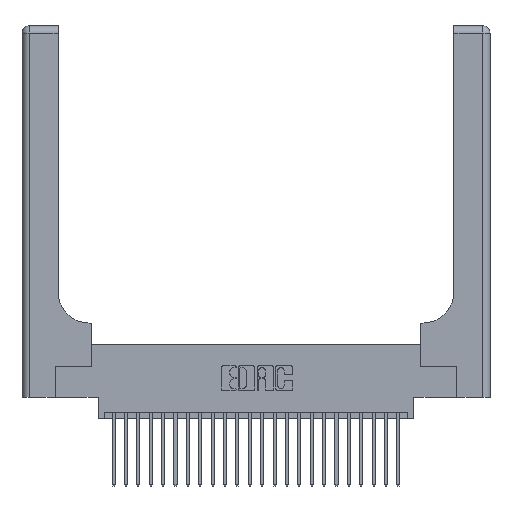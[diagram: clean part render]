
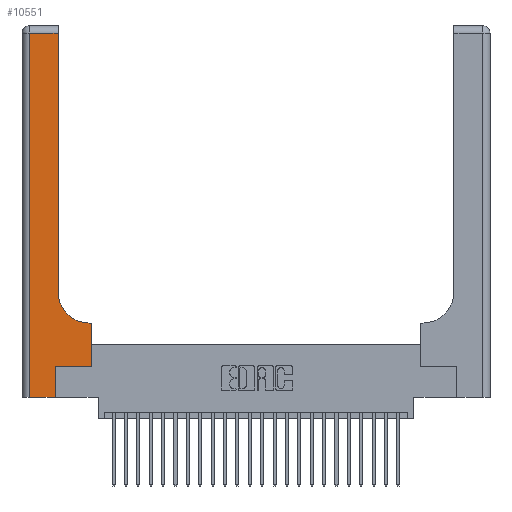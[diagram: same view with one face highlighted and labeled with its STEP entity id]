
A CAD part, top view. The second image highlights one B-rep face of the part: STEP entity #10551.
In plain terms, the highlighted planar face has unit normal (0, 0, 1).
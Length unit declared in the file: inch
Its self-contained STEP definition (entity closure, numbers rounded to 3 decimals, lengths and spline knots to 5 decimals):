
#645 = CARTESIAN_POINT ( 'NONE',  ( 0.5415, 0.6, 0.37 ) ) ;
#1730 = DIRECTION ( 'NONE',  ( 1., 0., 0. ) ) ;
#1792 = EDGE_CURVE ( 'NONE', #12622, #19311, #15619, .T. ) ;
#1806 = CARTESIAN_POINT ( 'NONE',  ( 0.269, 0., 0.37 ) ) ;
#1993 = AXIS2_PLACEMENT_3D ( 'NONE', #2356, #4441, #6528 ) ;
#2032 = EDGE_CURVE ( 'NONE', #14648, #12622, #22652, .T. ) ;
#2356 = CARTESIAN_POINT ( 'NONE',  ( 0., 3., 0.37 ) ) ;
#2486 = CARTESIAN_POINT ( 'NONE',  ( 0.5585, 0.25, 0.37 ) ) ;
#2696 = ORIENTED_EDGE ( 'NONE', *, *, #10886, .T. ) ;
#2832 = VECTOR ( 'NONE', #23845, 39.37008 ) ;
#3479 = ORIENTED_EDGE ( 'NONE', *, *, #20768, .T. ) ;
#4388 = DIRECTION ( 'NONE',  ( 0., 1., 0. ) ) ;
#4400 = LINE ( 'NONE', #2486, #14685 ) ;
#4441 = DIRECTION ( 'NONE',  ( 0., 0., -1. ) ) ;
#5413 = LINE ( 'NONE', #23519, #19540 ) ;
#5454 = CARTESIAN_POINT ( 'NONE',  ( 0., 2.94, 0.37 ) ) ;
#5510 = CARTESIAN_POINT ( 'NONE',  ( 0.06, 3., 0.37 ) ) ;
#6135 = EDGE_CURVE ( 'NONE', #19050, #14648, #14693, .T. ) ;
#6237 = EDGE_CURVE ( 'NONE', #21643, #13369, #22111, .T. ) ;
#6274 = CARTESIAN_POINT ( 'NONE',  ( 0.5585, 0.25, 0.37 ) ) ;
#6528 = DIRECTION ( 'NONE',  ( -1., 0., 0. ) ) ;
#6707 = FACE_OUTER_BOUND ( 'NONE', #12043, .T. ) ;
#7758 = EDGE_CURVE ( 'NONE', #13369, #19478, #13233, .T. ) ;
#8484 = LINE ( 'NONE', #5510, #23910 ) ;
#8554 = CARTESIAN_POINT ( 'NONE',  ( 0.2915, 2.94, 0.37 ) ) ;
#8697 = CARTESIAN_POINT ( 'NONE',  ( 0.5585, 0.6, 0.37 ) ) ;
#10245 = ORIENTED_EDGE ( 'NONE', *, *, #6135, .T. ) ;
#10497 = CARTESIAN_POINT ( 'NONE',  ( 0.06, 0., 0.37 ) ) ;
#10551 = ADVANCED_FACE ( 'NONE', ( #6707 ), #24910, .F. ) ;
#10886 = EDGE_CURVE ( 'NONE', #19478, #14336, #5413, .T. ) ;
#12017 = ORIENTED_EDGE ( 'NONE', *, *, #7758, .T. ) ;
#12043 = EDGE_LOOP ( 'NONE', ( #18715, #23758, #25726, #20669, #12017, #2696, #3479, #10245, #17749 ) ) ;
#12333 = CARTESIAN_POINT ( 'NONE',  ( 0.269, 0.25, 0.37 ) ) ;
#12622 = VERTEX_POINT ( 'NONE', #13863 ) ;
#12781 = DIRECTION ( 'NONE',  ( -1., 0., 0. ) ) ;
#12875 = CARTESIAN_POINT ( 'NONE',  ( 0.2915, 0.6, 0.37 ) ) ;
#13233 = LINE ( 'NONE', #1806, #16434 ) ;
#13369 = VERTEX_POINT ( 'NONE', #13397 ) ;
#13392 = EDGE_CURVE ( 'NONE', #20878, #21643, #8484, .T. ) ;
#13397 = CARTESIAN_POINT ( 'NONE',  ( 0.269, 0., 0.37 ) ) ;
#13863 = CARTESIAN_POINT ( 'NONE',  ( 0.2915, 0.85, 0.37 ) ) ;
#13911 = DIRECTION ( 'NONE',  ( 0., 1., 0. ) ) ;
#14336 = VERTEX_POINT ( 'NONE', #6274 ) ;
#14648 = VERTEX_POINT ( 'NONE', #645 ) ;
#14685 = VECTOR ( 'NONE', #4388, 39.37008 ) ;
#14693 = LINE ( 'NONE', #12875, #16000 ) ;
#15175 = DIRECTION ( 'NONE',  ( 0., 0., -1. ) ) ;
#15318 = CARTESIAN_POINT ( 'NONE',  ( 0., 0., 0.37 ) ) ;
#15449 = CARTESIAN_POINT ( 'NONE',  ( 0.06, 2.94, 0.37 ) ) ;
#15619 = LINE ( 'NONE', #17955, #25886 ) ;
#15639 = LINE ( 'NONE', #5454, #20754 ) ;
#16000 = VECTOR ( 'NONE', #12781, 39.37008 ) ;
#16136 = DIRECTION ( 'NONE',  ( 0., -1., 0. ) ) ;
#16434 = VECTOR ( 'NONE', #13911, 39.37008 ) ;
#17017 = EDGE_CURVE ( 'NONE', #19311, #20878, #15639, .T. ) ;
#17749 = ORIENTED_EDGE ( 'NONE', *, *, #2032, .T. ) ;
#17955 = CARTESIAN_POINT ( 'NONE',  ( 0.2915, 3., 0.37 ) ) ;
#18040 = DIRECTION ( 'NONE',  ( 0., 1., 0. ) ) ;
#18715 = ORIENTED_EDGE ( 'NONE', *, *, #1792, .T. ) ;
#19050 = VERTEX_POINT ( 'NONE', #8697 ) ;
#19311 = VERTEX_POINT ( 'NONE', #8554 ) ;
#19478 = VERTEX_POINT ( 'NONE', #12333 ) ;
#19540 = VECTOR ( 'NONE', #1730, 39.37008 ) ;
#20669 = ORIENTED_EDGE ( 'NONE', *, *, #6237, .T. ) ;
#20754 = VECTOR ( 'NONE', #21861, 39.37008 ) ;
#20768 = EDGE_CURVE ( 'NONE', #14336, #19050, #4400, .T. ) ;
#20878 = VERTEX_POINT ( 'NONE', #15449 ) ;
#21174 = CARTESIAN_POINT ( 'NONE',  ( 0.5415, 0.85, 0.37 ) ) ;
#21453 = DIRECTION ( 'NONE',  ( 1., 0., 0. ) ) ;
#21643 = VERTEX_POINT ( 'NONE', #10497 ) ;
#21861 = DIRECTION ( 'NONE',  ( -1., 0., 0. ) ) ;
#22111 = LINE ( 'NONE', #15318, #2832 ) ;
#22652 = CIRCLE ( 'NONE', #24284, 0.25 ) ;
#23519 = CARTESIAN_POINT ( 'NONE',  ( 0.269, 0.25, 0.37 ) ) ;
#23758 = ORIENTED_EDGE ( 'NONE', *, *, #17017, .T. ) ;
#23845 = DIRECTION ( 'NONE',  ( 1., 0., 0. ) ) ;
#23910 = VECTOR ( 'NONE', #16136, 39.37008 ) ;
#24284 = AXIS2_PLACEMENT_3D ( 'NONE', #21174, #15175, #21453 ) ;
#24910 = PLANE ( 'NONE',  #1993 ) ;
#25726 = ORIENTED_EDGE ( 'NONE', *, *, #13392, .T. ) ;
#25886 = VECTOR ( 'NONE', #18040, 39.37008 ) ;
